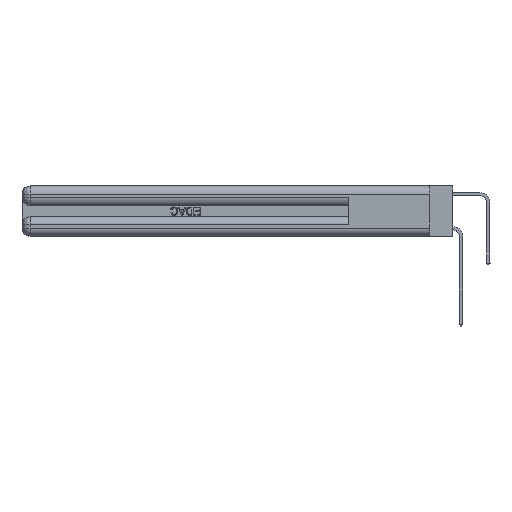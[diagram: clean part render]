
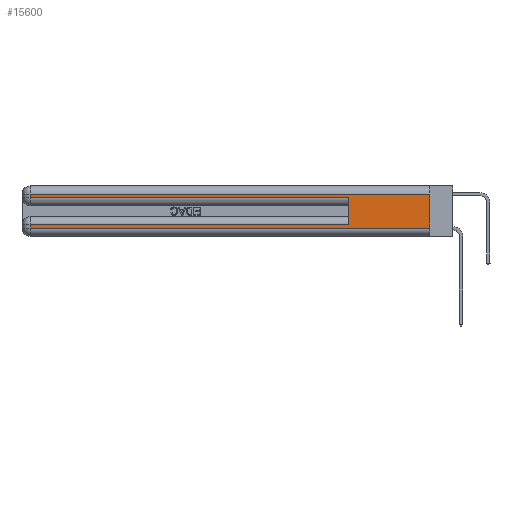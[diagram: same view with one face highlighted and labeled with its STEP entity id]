
A CAD part, left-side view. The second image highlights one B-rep face of the part: STEP entity #15600.
In plain terms, the highlighted planar face has unit normal (-1, 0, 0).
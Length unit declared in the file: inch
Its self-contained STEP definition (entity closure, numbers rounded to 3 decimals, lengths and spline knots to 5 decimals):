
#266 = EDGE_CURVE ( 'NONE', #7421, #32629, #16732, .T. ) ;
#604 = ORIENTED_EDGE ( 'NONE', *, *, #13692, .T. ) ;
#1022 = CARTESIAN_POINT ( 'NONE',  ( 0., 0., 0.37 ) ) ;
#1551 = VECTOR ( 'NONE', #1902, 39.37008 ) ;
#1902 = DIRECTION ( 'NONE',  ( 0., 0., -1. ) ) ;
#3158 = VERTEX_POINT ( 'NONE', #29019 ) ;
#3484 = DIRECTION ( 'NONE',  ( 0., -1., 0. ) ) ;
#3632 = DIRECTION ( 'NONE',  ( 1., 0., 0. ) ) ;
#4097 = VECTOR ( 'NONE', #6387, 39.37008 ) ;
#4709 = VECTOR ( 'NONE', #26496, 39.37008 ) ;
#5446 = DIRECTION ( 'NONE',  ( 0., 1., 0. ) ) ;
#5764 = ORIENTED_EDGE ( 'NONE', *, *, #5842, .T. ) ;
#5813 = LINE ( 'NONE', #19435, #32477 ) ;
#5842 = EDGE_CURVE ( 'NONE', #18165, #33440, #28746, .T. ) ;
#6387 = DIRECTION ( 'NONE',  ( 0., 1., 0. ) ) ;
#6805 = ORIENTED_EDGE ( 'NONE', *, *, #266, .T. ) ;
#7202 = VERTEX_POINT ( 'NONE', #22102 ) ;
#7421 = VERTEX_POINT ( 'NONE', #17897 ) ;
#9027 = FACE_OUTER_BOUND ( 'NONE', #26493, .T. ) ;
#9677 = VECTOR ( 'NONE', #5446, 39.37008 ) ;
#9775 = AXIS2_PLACEMENT_3D ( 'NONE', #1022, #3632, #30150 ) ;
#10197 = EDGE_CURVE ( 'NONE', #7202, #32629, #5813, .T. ) ;
#10225 = CARTESIAN_POINT ( 'NONE',  ( 0., 0., 0.285 ) ) ;
#11926 = VECTOR ( 'NONE', #18167, 39.37008 ) ;
#12769 = ORIENTED_EDGE ( 'NONE', *, *, #33465, .T. ) ;
#12875 = CARTESIAN_POINT ( 'NONE',  ( 0., 0.6, 0.285 ) ) ;
#12953 = EDGE_CURVE ( 'NONE', #25711, #3158, #33116, .T. ) ;
#13692 = EDGE_CURVE ( 'NONE', #7202, #26237, #26907, .T. ) ;
#14015 = EDGE_CURVE ( 'NONE', #25711, #33440, #23054, .T. ) ;
#14865 = CARTESIAN_POINT ( 'NONE',  ( 0., 0.6, 0.085 ) ) ;
#15435 = VECTOR ( 'NONE', #20875, 39.37008 ) ;
#15510 = LINE ( 'NONE', #34192, #4709 ) ;
#15600 = ADVANCED_FACE ( 'NONE', ( #9027 ), #19677, .F. ) ;
#16732 = LINE ( 'NONE', #16914, #30587 ) ;
#16914 = CARTESIAN_POINT ( 'NONE',  ( 0., 0., 0.06 ) ) ;
#17671 = ORIENTED_EDGE ( 'NONE', *, *, #19936, .T. ) ;
#17748 = CARTESIAN_POINT ( 'NONE',  ( 0., 2.94, 0.37 ) ) ;
#17897 = CARTESIAN_POINT ( 'NONE',  ( 0., 2.94, 0.06 ) ) ;
#18165 = VERTEX_POINT ( 'NONE', #18308 ) ;
#18167 = DIRECTION ( 'NONE',  ( 0., 0., 1. ) ) ;
#18308 = CARTESIAN_POINT ( 'NONE',  ( 0., 2.94, 0.285 ) ) ;
#19435 = CARTESIAN_POINT ( 'NONE',  ( 0., 0., 0.37 ) ) ;
#19677 = PLANE ( 'NONE',  #9775 ) ;
#19841 = CARTESIAN_POINT ( 'NONE',  ( 0., 0., 0.085 ) ) ;
#19936 = EDGE_CURVE ( 'NONE', #26237, #18165, #22815, .T. ) ;
#20875 = DIRECTION ( 'NONE',  ( 0., -1., 0. ) ) ;
#22102 = CARTESIAN_POINT ( 'NONE',  ( 0., 0., 0.31 ) ) ;
#22154 = CARTESIAN_POINT ( 'NONE',  ( 0., 2.94, 0.31 ) ) ;
#22815 = LINE ( 'NONE', #17748, #1551 ) ;
#23054 = LINE ( 'NONE', #31610, #11926 ) ;
#23561 = ORIENTED_EDGE ( 'NONE', *, *, #14015, .F. ) ;
#25711 = VERTEX_POINT ( 'NONE', #14865 ) ;
#26237 = VERTEX_POINT ( 'NONE', #22154 ) ;
#26493 = EDGE_LOOP ( 'NONE', ( #28141, #604, #17671, #5764, #23561, #26548, #12769, #6805 ) ) ;
#26496 = DIRECTION ( 'NONE',  ( 0., 0., -1. ) ) ;
#26548 = ORIENTED_EDGE ( 'NONE', *, *, #12953, .T. ) ;
#26907 = LINE ( 'NONE', #32342, #9677 ) ;
#27459 = DIRECTION ( 'NONE',  ( 0., 0., -1. ) ) ;
#28141 = ORIENTED_EDGE ( 'NONE', *, *, #10197, .F. ) ;
#28746 = LINE ( 'NONE', #10225, #15435 ) ;
#29019 = CARTESIAN_POINT ( 'NONE',  ( 0., 2.94, 0.085 ) ) ;
#30150 = DIRECTION ( 'NONE',  ( 0., 0., -1. ) ) ;
#30241 = CARTESIAN_POINT ( 'NONE',  ( 0., 0., 0.06 ) ) ;
#30587 = VECTOR ( 'NONE', #3484, 39.37008 ) ;
#31610 = CARTESIAN_POINT ( 'NONE',  ( 0., 0.6, 0.145 ) ) ;
#32342 = CARTESIAN_POINT ( 'NONE',  ( 0., 0., 0.31 ) ) ;
#32477 = VECTOR ( 'NONE', #27459, 39.37008 ) ;
#32629 = VERTEX_POINT ( 'NONE', #30241 ) ;
#33116 = LINE ( 'NONE', #19841, #4097 ) ;
#33440 = VERTEX_POINT ( 'NONE', #12875 ) ;
#33465 = EDGE_CURVE ( 'NONE', #3158, #7421, #15510, .T. ) ;
#34192 = CARTESIAN_POINT ( 'NONE',  ( 0., 2.94, 0.37 ) ) ;
